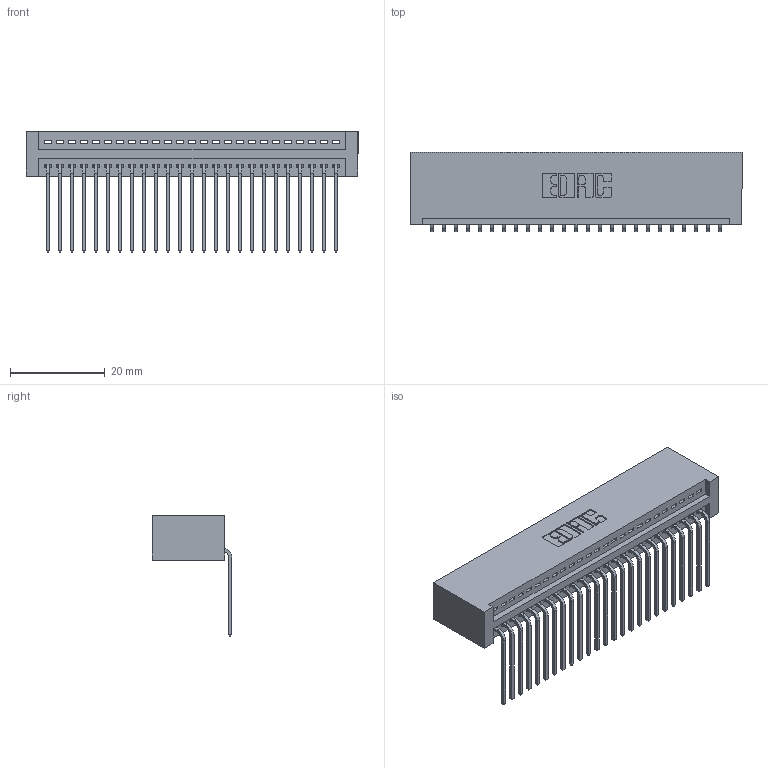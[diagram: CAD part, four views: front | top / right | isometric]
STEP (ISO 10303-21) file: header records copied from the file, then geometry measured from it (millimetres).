
FILE_DESCRIPTION (( 'STEP AP203' ), '1' );
FILE_NAME ('395-025-559-101.STEP', '2019-10-18T08:31:36', ( '' ), ( '' ), 'SwSTEP 2.0', 'SolidWorks 2016', '' );
FILE_SCHEMA (( 'CONFIG_CONTROL_DESIGN' ));
Length unit declared in the file: inch
Products named in the file (3): 345-292-001_558 559 Tail - 1; 345 Part_No Mounting Lugs; 395-025-559-101
Assembly tree (26 placements, depth 2):
  395-025-559-101
    345 Part_No Mounting Lugs
    345-292-001_558 559 Tail - 1  x25
Bounding box: 70.1 x 16.75 x 25.53 mm (x, y, z)
Volume: 7186.9 mm3; surface area: 9999.3 mm2
Topology: 26 solids, 26 shells, 1618 faces, 4867 edges, 3210 vertices
Faces by surface type: plane 1126, cylinder 492
Entity records: 20911 total; most frequent: CARTESIAN_POINT 3631, ORIENTED_EDGE 3590, DIRECTION 3189, EDGE_CURVE 1795, VECTOR 1571, LINE 1571, VERTEX_POINT 1194, AXIS2_PLACEMENT_3D 809
